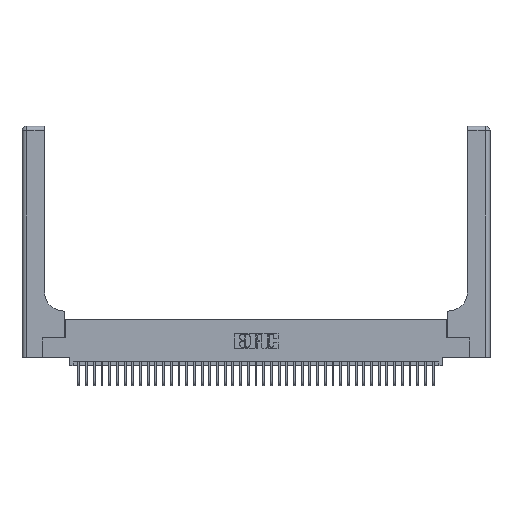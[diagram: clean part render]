
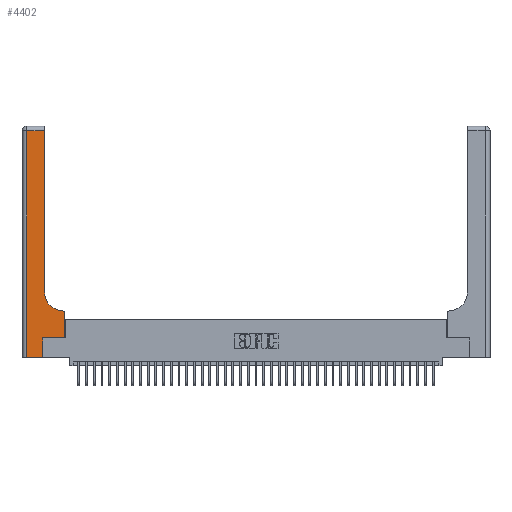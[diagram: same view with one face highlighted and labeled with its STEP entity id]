
A CAD part, top view. The second image highlights one B-rep face of the part: STEP entity #4402.
In plain terms, the highlighted planar face has unit normal (0, 0, 1).
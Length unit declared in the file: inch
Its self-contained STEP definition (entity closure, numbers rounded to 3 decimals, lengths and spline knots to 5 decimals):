
#388 = FACE_OUTER_BOUND ( 'NONE', #32698, .T. ) ;
#1359 = EDGE_CURVE ( 'NONE', #19723, #35424, #15893, .T. ) ;
#2157 = VERTEX_POINT ( 'NONE', #8211 ) ;
#2602 = DIRECTION ( 'NONE',  ( 0., 1., 0. ) ) ;
#2805 = LINE ( 'NONE', #22757, #33748 ) ;
#2828 = DIRECTION ( 'NONE',  ( 0., 1., 0. ) ) ;
#2929 = DIRECTION ( 'NONE',  ( 1., 0., 0. ) ) ;
#3125 = EDGE_CURVE ( 'NONE', #36290, #2157, #29517, .T. ) ;
#3650 = CARTESIAN_POINT ( 'NONE',  ( 0.5585, 0.25, 0.37 ) ) ;
#4402 = ADVANCED_FACE ( 'NONE', ( #388 ), #35630, .F. ) ;
#5838 = CARTESIAN_POINT ( 'NONE',  ( 0., 0., 0.37 ) ) ;
#6941 = CARTESIAN_POINT ( 'NONE',  ( 0.2915, 2.94, 0.37 ) ) ;
#7301 = CARTESIAN_POINT ( 'NONE',  ( 0.269, 0., 0.37 ) ) ;
#7538 = EDGE_CURVE ( 'NONE', #23706, #36134, #15172, .T. ) ;
#7902 = DIRECTION ( 'NONE',  ( -1., 0., 0. ) ) ;
#7981 = LINE ( 'NONE', #39915, #15203 ) ;
#8211 = CARTESIAN_POINT ( 'NONE',  ( 0.5585, 0.6, 0.37 ) ) ;
#9458 = ORIENTED_EDGE ( 'NONE', *, *, #39501, .T. ) ;
#9506 = DIRECTION ( 'NONE',  ( 1., 0., 0. ) ) ;
#11124 = CARTESIAN_POINT ( 'NONE',  ( 0.5415, 0.6, 0.37 ) ) ;
#11523 = DIRECTION ( 'NONE',  ( 1., 0., 0. ) ) ;
#12170 = ORIENTED_EDGE ( 'NONE', *, *, #39412, .T. ) ;
#12718 = AXIS2_PLACEMENT_3D ( 'NONE', #40007, #21381, #2929 ) ;
#12805 = CARTESIAN_POINT ( 'NONE',  ( 0.2915, 0.85, 0.37 ) ) ;
#12848 = ORIENTED_EDGE ( 'NONE', *, *, #1359, .T. ) ;
#13636 = DIRECTION ( 'NONE',  ( -1., 0., 0. ) ) ;
#13867 = VERTEX_POINT ( 'NONE', #11124 ) ;
#14884 = CARTESIAN_POINT ( 'NONE',  ( 0.269, 0., 0.37 ) ) ;
#14942 = VECTOR ( 'NONE', #2828, 39.37008 ) ;
#15172 = LINE ( 'NONE', #5838, #31637 ) ;
#15203 = VECTOR ( 'NONE', #24416, 39.37008 ) ;
#15893 = LINE ( 'NONE', #27522, #14942 ) ;
#16092 = CIRCLE ( 'NONE', #12718, 0.25 ) ;
#16620 = ORIENTED_EDGE ( 'NONE', *, *, #3125, .T. ) ;
#17452 = CARTESIAN_POINT ( 'NONE',  ( 0.06, 0., 0.37 ) ) ;
#18238 = DIRECTION ( 'NONE',  ( -1., 0., 0. ) ) ;
#19723 = VERTEX_POINT ( 'NONE', #12805 ) ;
#20134 = CARTESIAN_POINT ( 'NONE',  ( 0., 3., 0.37 ) ) ;
#20493 = ORIENTED_EDGE ( 'NONE', *, *, #36156, .T. ) ;
#20813 = EDGE_CURVE ( 'NONE', #36134, #37870, #31569, .T. ) ;
#21075 = CARTESIAN_POINT ( 'NONE',  ( 0.06, 2.94, 0.37 ) ) ;
#21381 = DIRECTION ( 'NONE',  ( 0., 0., -1. ) ) ;
#21592 = AXIS2_PLACEMENT_3D ( 'NONE', #20134, #26360, #7902 ) ;
#21701 = CARTESIAN_POINT ( 'NONE',  ( 0.269, 0.25, 0.37 ) ) ;
#22091 = DIRECTION ( 'NONE',  ( 0., 1., 0. ) ) ;
#22130 = LINE ( 'NONE', #21701, #37738 ) ;
#22757 = CARTESIAN_POINT ( 'NONE',  ( 0.2915, 0.6, 0.37 ) ) ;
#23389 = CARTESIAN_POINT ( 'NONE',  ( 0.269, 0.25, 0.37 ) ) ;
#23706 = VERTEX_POINT ( 'NONE', #17452 ) ;
#24416 = DIRECTION ( 'NONE',  ( 0., -1., 0. ) ) ;
#26054 = VECTOR ( 'NONE', #18238, 39.37008 ) ;
#26360 = DIRECTION ( 'NONE',  ( 0., 0., -1. ) ) ;
#26778 = EDGE_CURVE ( 'NONE', #13867, #19723, #16092, .T. ) ;
#27370 = ORIENTED_EDGE ( 'NONE', *, *, #7538, .T. ) ;
#27390 = VERTEX_POINT ( 'NONE', #21075 ) ;
#27522 = CARTESIAN_POINT ( 'NONE',  ( 0.2915, 3., 0.37 ) ) ;
#29517 = LINE ( 'NONE', #3650, #37800 ) ;
#30580 = VECTOR ( 'NONE', #2602, 39.37008 ) ;
#31406 = ORIENTED_EDGE ( 'NONE', *, *, #38698, .T. ) ;
#31569 = LINE ( 'NONE', #14884, #30580 ) ;
#31637 = VECTOR ( 'NONE', #11523, 39.37008 ) ;
#31731 = ORIENTED_EDGE ( 'NONE', *, *, #20813, .T. ) ;
#32698 = EDGE_LOOP ( 'NONE', ( #12848, #12170, #31406, #27370, #31731, #9458, #16620, #20493, #34259 ) ) ;
#33748 = VECTOR ( 'NONE', #13636, 39.37008 ) ;
#34259 = ORIENTED_EDGE ( 'NONE', *, *, #26778, .T. ) ;
#34324 = LINE ( 'NONE', #36839, #26054 ) ;
#35424 = VERTEX_POINT ( 'NONE', #6941 ) ;
#35630 = PLANE ( 'NONE',  #21592 ) ;
#36134 = VERTEX_POINT ( 'NONE', #7301 ) ;
#36156 = EDGE_CURVE ( 'NONE', #2157, #13867, #2805, .T. ) ;
#36290 = VERTEX_POINT ( 'NONE', #40078 ) ;
#36839 = CARTESIAN_POINT ( 'NONE',  ( 0., 2.94, 0.37 ) ) ;
#37738 = VECTOR ( 'NONE', #9506, 39.37008 ) ;
#37800 = VECTOR ( 'NONE', #22091, 39.37008 ) ;
#37870 = VERTEX_POINT ( 'NONE', #23389 ) ;
#38698 = EDGE_CURVE ( 'NONE', #27390, #23706, #7981, .T. ) ;
#39412 = EDGE_CURVE ( 'NONE', #35424, #27390, #34324, .T. ) ;
#39501 = EDGE_CURVE ( 'NONE', #37870, #36290, #22130, .T. ) ;
#39915 = CARTESIAN_POINT ( 'NONE',  ( 0.06, 3., 0.37 ) ) ;
#40007 = CARTESIAN_POINT ( 'NONE',  ( 0.5415, 0.85, 0.37 ) ) ;
#40078 = CARTESIAN_POINT ( 'NONE',  ( 0.5585, 0.25, 0.37 ) ) ;
